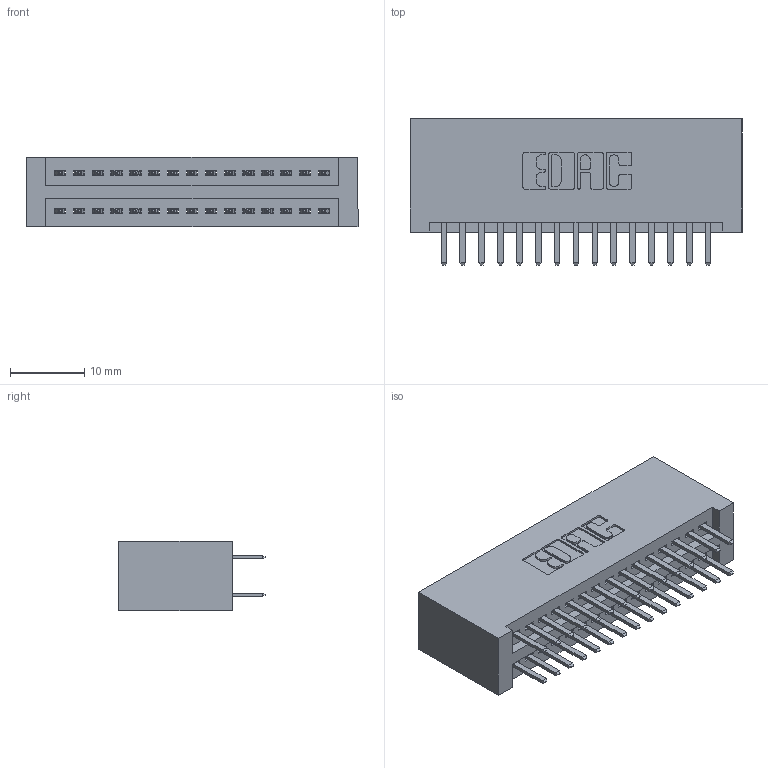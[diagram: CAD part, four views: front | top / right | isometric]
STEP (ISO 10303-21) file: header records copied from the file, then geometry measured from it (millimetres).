
FILE_DESCRIPTION (( 'STEP AP203' ), '1' );
FILE_NAME ('395-030-520-201.STEP', '2018-11-10T22:20:27', ( '' ), ( '' ), 'SwSTEP 2.0', 'SolidWorks 2016', '' );
FILE_SCHEMA (( 'CONFIG_CONTROL_DESIGN' ));
Length unit declared in the file: inch
Products named in the file (3): 395-030-520-201; 345 Part_No Mounting Lugs; 345-292-001_345-293-120
Assembly tree (31 placements, depth 2):
  395-030-520-201
    345 Part_No Mounting Lugs
    345-292-001_345-293-120  x30
Bounding box: 44.7 x 19.68 x 9.4 mm (x, y, z)
Volume: 4694.7 mm3; surface area: 6691.8 mm2
Topology: 31 solids, 31 shells, 1738 faces, 5027 edges, 3270 vertices
Faces by surface type: plane 1126, cylinder 612
Entity records: 15241 total; most frequent: CARTESIAN_POINT 2592, ORIENTED_EDGE 2514, DIRECTION 2301, EDGE_CURVE 1257, VECTOR 1069, LINE 1069, VERTEX_POINT 834, AXIS2_PLACEMENT_3D 616
